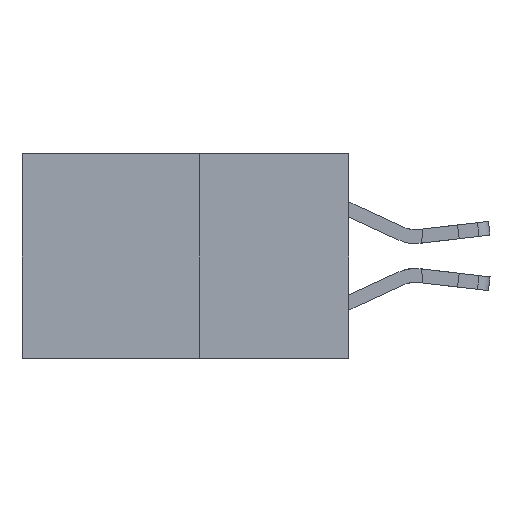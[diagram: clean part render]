
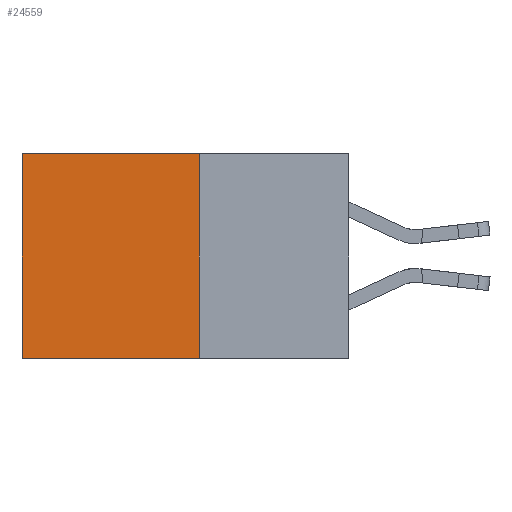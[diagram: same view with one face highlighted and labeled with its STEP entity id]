
A CAD part, left-side view. The second image highlights one B-rep face of the part: STEP entity #24559.
In plain terms, the highlighted planar face has unit normal (-1, 0, 0).
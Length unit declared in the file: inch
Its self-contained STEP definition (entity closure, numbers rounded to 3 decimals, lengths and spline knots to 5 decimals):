
#645 = EDGE_CURVE ( 'NONE', #19509, #1247, #18667, .T. ) ;
#1247 = VERTEX_POINT ( 'NONE', #3900 ) ;
#2977 = VECTOR ( 'NONE', #22590, 39.37008 ) ;
#3900 = CARTESIAN_POINT ( 'NONE',  ( 0.277, 0.59, 0. ) ) ;
#5371 = VERTEX_POINT ( 'NONE', #5517 ) ;
#5517 = CARTESIAN_POINT ( 'NONE',  ( 0.277, 0.59, -0.37 ) ) ;
#6401 = VECTOR ( 'NONE', #17985, 39.37008 ) ;
#7011 = VECTOR ( 'NONE', #11022, 39.37008 ) ;
#7041 = LINE ( 'NONE', #25937, #6401 ) ;
#7493 = ORIENTED_EDGE ( 'NONE', *, *, #645, .T. ) ;
#7715 = CARTESIAN_POINT ( 'NONE',  ( 0.277, 0.27, 0. ) ) ;
#7758 = LINE ( 'NONE', #11586, #18037 ) ;
#9288 = EDGE_CURVE ( 'NONE', #19509, #10806, #7758, .T. ) ;
#9762 = AXIS2_PLACEMENT_3D ( 'NONE', #23232, #23322, #11158 ) ;
#10680 = EDGE_CURVE ( 'NONE', #10806, #5371, #7041, .T. ) ;
#10806 = VERTEX_POINT ( 'NONE', #16342 ) ;
#11022 = DIRECTION ( 'NONE',  ( 0., 0., -1. ) ) ;
#11158 = DIRECTION ( 'NONE',  ( 0., 0., -1. ) ) ;
#11586 = CARTESIAN_POINT ( 'NONE',  ( 0.277, 0.27, -0.37 ) ) ;
#11837 = LINE ( 'NONE', #23181, #7011 ) ;
#11886 = ORIENTED_EDGE ( 'NONE', *, *, #9288, .F. ) ;
#12087 = EDGE_LOOP ( 'NONE', ( #23343, #17428, #11886, #7493 ) ) ;
#15719 = DIRECTION ( 'NONE',  ( 0., 0., -1. ) ) ;
#16288 = FACE_OUTER_BOUND ( 'NONE', #12087, .T. ) ;
#16342 = CARTESIAN_POINT ( 'NONE',  ( 0.277, 0.27, -0.37 ) ) ;
#17428 = ORIENTED_EDGE ( 'NONE', *, *, #10680, .F. ) ;
#17985 = DIRECTION ( 'NONE',  ( 0., 1., 0. ) ) ;
#18037 = VECTOR ( 'NONE', #15719, 39.37008 ) ;
#18667 = LINE ( 'NONE', #7715, #2977 ) ;
#18884 = EDGE_CURVE ( 'NONE', #1247, #5371, #11837, .T. ) ;
#19313 = PLANE ( 'NONE',  #9762 ) ;
#19509 = VERTEX_POINT ( 'NONE', #24886 ) ;
#22590 = DIRECTION ( 'NONE',  ( 0., 1., 0. ) ) ;
#23181 = CARTESIAN_POINT ( 'NONE',  ( 0.277, 0.59, -0.37 ) ) ;
#23232 = CARTESIAN_POINT ( 'NONE',  ( 0.277, 0.27, -0.37 ) ) ;
#23322 = DIRECTION ( 'NONE',  ( 1., 0., 0. ) ) ;
#23343 = ORIENTED_EDGE ( 'NONE', *, *, #18884, .T. ) ;
#24559 = ADVANCED_FACE ( 'NONE', ( #16288 ), #19313, .F. ) ;
#24886 = CARTESIAN_POINT ( 'NONE',  ( 0.277, 0.27, 0. ) ) ;
#25937 = CARTESIAN_POINT ( 'NONE',  ( 0.277, 0.27, -0.37 ) ) ;
